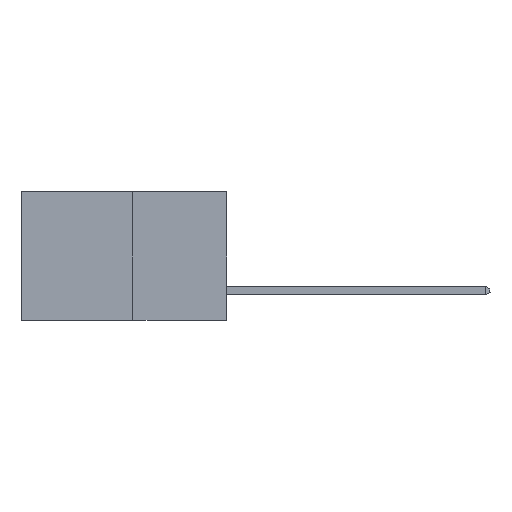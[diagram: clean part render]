
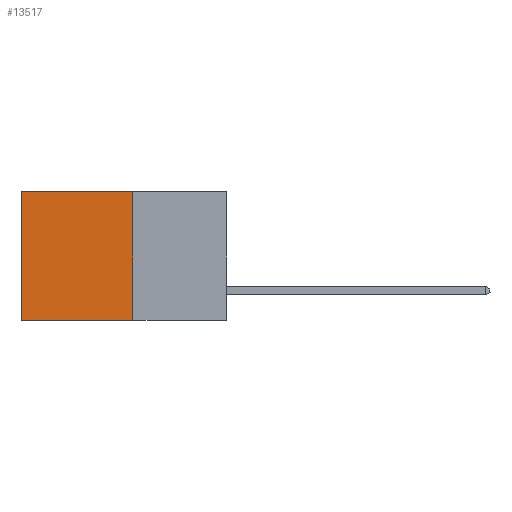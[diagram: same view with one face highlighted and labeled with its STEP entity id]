
A CAD part, left-side view. The second image highlights one B-rep face of the part: STEP entity #13517.
In plain terms, the highlighted planar face has unit normal (-1, 0, 0).
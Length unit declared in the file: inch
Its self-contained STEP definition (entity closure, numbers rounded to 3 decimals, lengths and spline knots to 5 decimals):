
#1104 = VECTOR ( 'NONE', #31603, 39.37008 ) ;
#2478 = PLANE ( 'NONE',  #27945 ) ;
#3454 = VECTOR ( 'NONE', #12516, 39.37008 ) ;
#4689 = CARTESIAN_POINT ( 'NONE',  ( 0.277, 0.27, -0.37 ) ) ;
#5014 = DIRECTION ( 'NONE',  ( 1., 0., 0. ) ) ;
#5304 = ORIENTED_EDGE ( 'NONE', *, *, #23227, .T. ) ;
#8581 = EDGE_CURVE ( 'NONE', #12407, #16465, #18045, .T. ) ;
#12377 = CARTESIAN_POINT ( 'NONE',  ( 0.277, 0.27, -0.37 ) ) ;
#12407 = VERTEX_POINT ( 'NONE', #18320 ) ;
#12516 = DIRECTION ( 'NONE',  ( 0., 1., 0. ) ) ;
#13517 = ADVANCED_FACE ( 'NONE', ( #30140 ), #2478, .F. ) ;
#13690 = LINE ( 'NONE', #16634, #1104 ) ;
#13966 = CARTESIAN_POINT ( 'NONE',  ( 0.277, 0.59, 0. ) ) ;
#15240 = CARTESIAN_POINT ( 'NONE',  ( 0.277, 0.59, -0.37 ) ) ;
#16465 = VERTEX_POINT ( 'NONE', #22737 ) ;
#16634 = CARTESIAN_POINT ( 'NONE',  ( 0.277, 0.27, -0.37 ) ) ;
#18045 = LINE ( 'NONE', #4689, #23912 ) ;
#18052 = ORIENTED_EDGE ( 'NONE', *, *, #8581, .F. ) ;
#18320 = CARTESIAN_POINT ( 'NONE',  ( 0.277, 0.27, -0.37 ) ) ;
#20031 = EDGE_CURVE ( 'NONE', #30281, #12407, #13690, .T. ) ;
#22643 = DIRECTION ( 'NONE',  ( 0., 0., -1. ) ) ;
#22737 = CARTESIAN_POINT ( 'NONE',  ( 0.277, 0.59, -0.37 ) ) ;
#23046 = EDGE_CURVE ( 'NONE', #30281, #28286, #23573, .T. ) ;
#23227 = EDGE_CURVE ( 'NONE', #28286, #16465, #32111, .T. ) ;
#23573 = LINE ( 'NONE', #29936, #3454 ) ;
#23711 = CARTESIAN_POINT ( 'NONE',  ( 0.277, 0.27, 0. ) ) ;
#23912 = VECTOR ( 'NONE', #24846, 39.37008 ) ;
#23944 = VECTOR ( 'NONE', #27765, 39.37008 ) ;
#24513 = ORIENTED_EDGE ( 'NONE', *, *, #23046, .T. ) ;
#24747 = EDGE_LOOP ( 'NONE', ( #5304, #18052, #32553, #24513 ) ) ;
#24846 = DIRECTION ( 'NONE',  ( 0., 1., 0. ) ) ;
#27765 = DIRECTION ( 'NONE',  ( 0., 0., -1. ) ) ;
#27945 = AXIS2_PLACEMENT_3D ( 'NONE', #12377, #5014, #22643 ) ;
#28286 = VERTEX_POINT ( 'NONE', #13966 ) ;
#29936 = CARTESIAN_POINT ( 'NONE',  ( 0.277, 0.27, 0. ) ) ;
#30140 = FACE_OUTER_BOUND ( 'NONE', #24747, .T. ) ;
#30281 = VERTEX_POINT ( 'NONE', #23711 ) ;
#31603 = DIRECTION ( 'NONE',  ( 0., 0., -1. ) ) ;
#32111 = LINE ( 'NONE', #15240, #23944 ) ;
#32553 = ORIENTED_EDGE ( 'NONE', *, *, #20031, .F. ) ;
